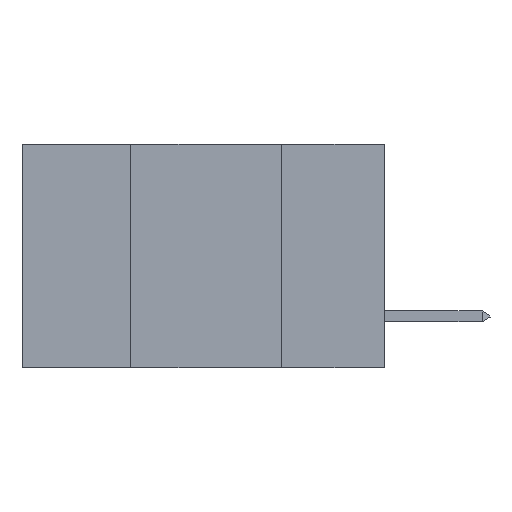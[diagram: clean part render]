
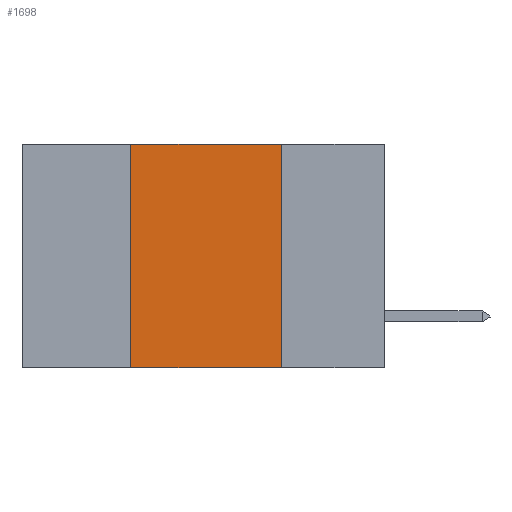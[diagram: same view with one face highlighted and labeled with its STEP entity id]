
A CAD part, left-side view. The second image highlights one B-rep face of the part: STEP entity #1698.
In plain terms, the highlighted planar face has unit normal (-1, 0, 0).
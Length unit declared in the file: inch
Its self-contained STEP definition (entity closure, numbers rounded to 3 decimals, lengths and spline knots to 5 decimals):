
#388 = EDGE_LOOP ( 'NONE', ( #3411, #5916, #1735, #3118 ) ) ;
#498 = VERTEX_POINT ( 'NONE', #6584 ) ;
#1180 = EDGE_CURVE ( 'NONE', #498, #3649, #4413, .T. ) ;
#1431 = EDGE_CURVE ( 'NONE', #498, #11254, #4188, .T. ) ;
#1698 = ADVANCED_FACE ( 'NONE', ( #16428 ), #6676, .F. ) ;
#1735 = ORIENTED_EDGE ( 'NONE', *, *, #1180, .F. ) ;
#2276 = DIRECTION ( 'NONE',  ( 0., 0., -1. ) ) ;
#2294 = VERTEX_POINT ( 'NONE', #16123 ) ;
#2873 = CARTESIAN_POINT ( 'NONE',  ( 0., 0.42, 0. ) ) ;
#2956 = DIRECTION ( 'NONE',  ( 0., 0., 1. ) ) ;
#3118 = ORIENTED_EDGE ( 'NONE', *, *, #1431, .T. ) ;
#3166 = CARTESIAN_POINT ( 'NONE',  ( 0., 0.6, 0. ) ) ;
#3411 = ORIENTED_EDGE ( 'NONE', *, *, #5305, .F. ) ;
#3649 = VERTEX_POINT ( 'NONE', #8291 ) ;
#4188 = LINE ( 'NONE', #11862, #13730 ) ;
#4413 = LINE ( 'NONE', #2873, #14349 ) ;
#5305 = EDGE_CURVE ( 'NONE', #2294, #11254, #14819, .T. ) ;
#5916 = ORIENTED_EDGE ( 'NONE', *, *, #6920, .F. ) ;
#6416 = DIRECTION ( 'NONE',  ( 0., 0., -1. ) ) ;
#6436 = DIRECTION ( 'NONE',  ( 1., 0., 0. ) ) ;
#6567 = CARTESIAN_POINT ( 'NONE',  ( 0., 0.17, -0.37 ) ) ;
#6584 = CARTESIAN_POINT ( 'NONE',  ( 0., 0.42, -0.37 ) ) ;
#6618 = CARTESIAN_POINT ( 'NONE',  ( 0., 0.6, 0. ) ) ;
#6676 = PLANE ( 'NONE',  #14153 ) ;
#6920 = EDGE_CURVE ( 'NONE', #3649, #2294, #15453, .T. ) ;
#8291 = CARTESIAN_POINT ( 'NONE',  ( 0., 0.42, 0. ) ) ;
#9803 = DIRECTION ( 'NONE',  ( 0., -1., 0. ) ) ;
#10219 = CARTESIAN_POINT ( 'NONE',  ( 0., 0.17, 0. ) ) ;
#11254 = VERTEX_POINT ( 'NONE', #6567 ) ;
#11374 = VECTOR ( 'NONE', #2276, 39.37008 ) ;
#11563 = DIRECTION ( 'NONE',  ( 0., -1., 0. ) ) ;
#11862 = CARTESIAN_POINT ( 'NONE',  ( 0., 0.6, -0.37 ) ) ;
#12069 = VECTOR ( 'NONE', #9803, 39.37008 ) ;
#13730 = VECTOR ( 'NONE', #11563, 39.37008 ) ;
#14153 = AXIS2_PLACEMENT_3D ( 'NONE', #6618, #6436, #6416 ) ;
#14349 = VECTOR ( 'NONE', #2956, 39.37008 ) ;
#14819 = LINE ( 'NONE', #10219, #11374 ) ;
#15453 = LINE ( 'NONE', #3166, #12069 ) ;
#16123 = CARTESIAN_POINT ( 'NONE',  ( 0., 0.17, 0. ) ) ;
#16428 = FACE_OUTER_BOUND ( 'NONE', #388, .T. ) ;
